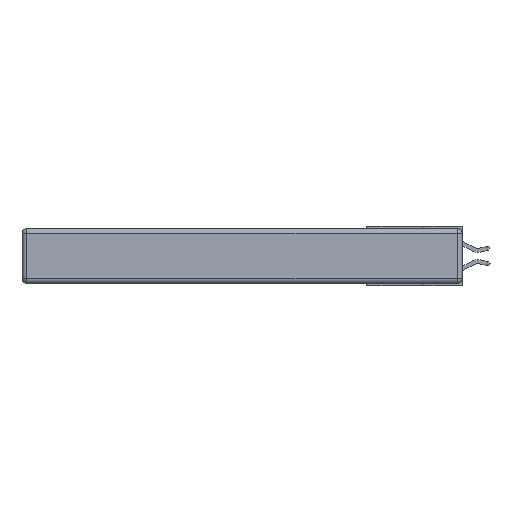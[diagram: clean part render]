
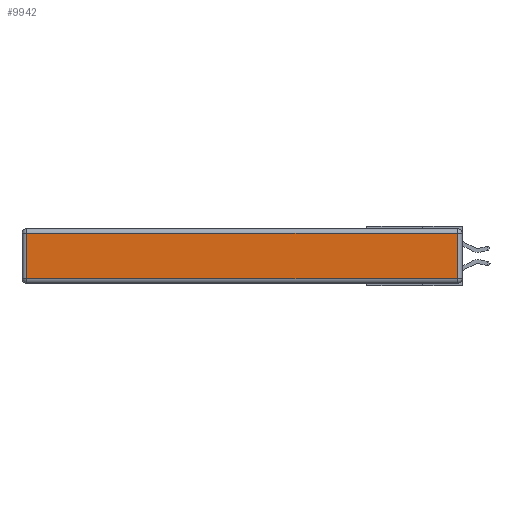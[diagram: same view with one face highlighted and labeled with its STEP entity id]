
A CAD part, left-side view. The second image highlights one B-rep face of the part: STEP entity #9942.
In plain terms, the highlighted planar face has unit normal (-1, 0, 0).
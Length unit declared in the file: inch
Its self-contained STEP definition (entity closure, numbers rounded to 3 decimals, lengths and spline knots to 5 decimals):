
#433 = LINE ( 'NONE', #5307, #8531 ) ;
#452 = CARTESIAN_POINT ( 'NONE',  ( 0., 0.03, -0.313 ) ) ;
#558 = ORIENTED_EDGE ( 'NONE', *, *, #14017, .T. ) ;
#1889 = CARTESIAN_POINT ( 'NONE',  ( 0., 2.72, -0.343 ) ) ;
#2917 = DIRECTION ( 'NONE',  ( 0., -1., 0. ) ) ;
#3006 = CARTESIAN_POINT ( 'NONE',  ( 0., 0., -0.343 ) ) ;
#3223 = AXIS2_PLACEMENT_3D ( 'NONE', #3006, #8328, #9426 ) ;
#3367 = VECTOR ( 'NONE', #7672, 39.37008 ) ;
#3528 = VECTOR ( 'NONE', #5173, 39.37008 ) ;
#4064 = CARTESIAN_POINT ( 'NONE',  ( 0., 2.75, -0.03 ) ) ;
#4133 = DIRECTION ( 'NONE',  ( 0., 0., -1. ) ) ;
#4718 = EDGE_LOOP ( 'NONE', ( #8939, #13750, #10568, #558 ) ) ;
#5145 = CARTESIAN_POINT ( 'NONE',  ( 0., 2.72, -0.313 ) ) ;
#5173 = DIRECTION ( 'NONE',  ( 0., 1., 0. ) ) ;
#5307 = CARTESIAN_POINT ( 'NONE',  ( 0., 0., -0.313 ) ) ;
#5699 = FACE_OUTER_BOUND ( 'NONE', #4718, .T. ) ;
#7045 = VERTEX_POINT ( 'NONE', #452 ) ;
#7672 = DIRECTION ( 'NONE',  ( 0., 0., 1. ) ) ;
#8328 = DIRECTION ( 'NONE',  ( -1., 0., 0. ) ) ;
#8531 = VECTOR ( 'NONE', #2917, 39.37008 ) ;
#8939 = ORIENTED_EDGE ( 'NONE', *, *, #13679, .T. ) ;
#9389 = LINE ( 'NONE', #4064, #3528 ) ;
#9426 = DIRECTION ( 'NONE',  ( 0., 0., 1. ) ) ;
#9509 = VERTEX_POINT ( 'NONE', #11895 ) ;
#9569 = PLANE ( 'NONE',  #3223 ) ;
#9942 = ADVANCED_FACE ( 'NONE', ( #5699 ), #9569, .T. ) ;
#10068 = CARTESIAN_POINT ( 'NONE',  ( 0., 0.03, -0.343 ) ) ;
#10395 = VECTOR ( 'NONE', #4133, 39.37008 ) ;
#10560 = VERTEX_POINT ( 'NONE', #5145 ) ;
#10568 = ORIENTED_EDGE ( 'NONE', *, *, #12486, .T. ) ;
#11125 = LINE ( 'NONE', #1889, #10395 ) ;
#11691 = CARTESIAN_POINT ( 'NONE',  ( 0., 2.72, -0.03 ) ) ;
#11895 = CARTESIAN_POINT ( 'NONE',  ( 0., 0.03, -0.03 ) ) ;
#12285 = EDGE_CURVE ( 'NONE', #7045, #9509, #12550, .T. ) ;
#12486 = EDGE_CURVE ( 'NONE', #9509, #12771, #9389, .T. ) ;
#12550 = LINE ( 'NONE', #10068, #3367 ) ;
#12771 = VERTEX_POINT ( 'NONE', #11691 ) ;
#13679 = EDGE_CURVE ( 'NONE', #10560, #7045, #433, .T. ) ;
#13750 = ORIENTED_EDGE ( 'NONE', *, *, #12285, .T. ) ;
#14017 = EDGE_CURVE ( 'NONE', #12771, #10560, #11125, .T. ) ;
